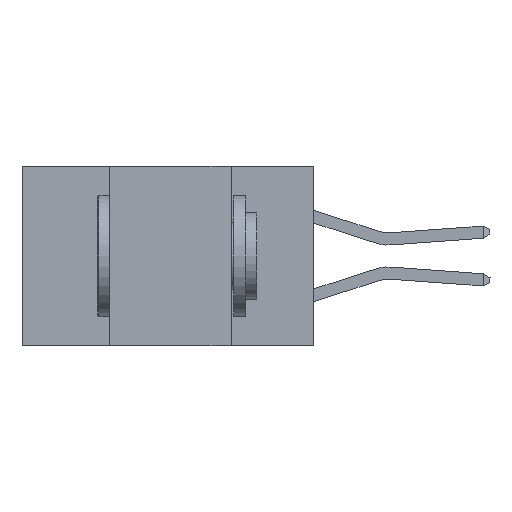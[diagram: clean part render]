
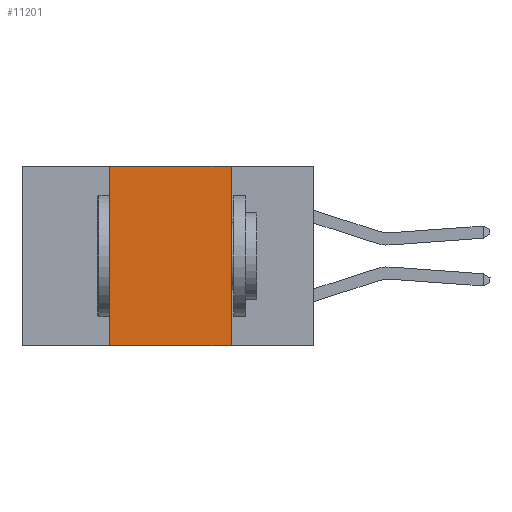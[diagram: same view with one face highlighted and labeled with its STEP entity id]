
A CAD part, left-side view. The second image highlights one B-rep face of the part: STEP entity #11201.
In plain terms, the highlighted planar face has unit normal (-1, 0, 0).
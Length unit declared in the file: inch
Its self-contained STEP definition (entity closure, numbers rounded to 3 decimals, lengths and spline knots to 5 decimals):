
#2424 = ORIENTED_EDGE ( 'NONE', *, *, #34790, .F. ) ;
#2858 = PLANE ( 'NONE',  #18497 ) ;
#3801 = ORIENTED_EDGE ( 'NONE', *, *, #26579, .F. ) ;
#4964 = LINE ( 'NONE', #28506, #28670 ) ;
#5660 = ORIENTED_EDGE ( 'NONE', *, *, #21838, .T. ) ;
#5968 = DIRECTION ( 'NONE',  ( 1., 0., 0. ) ) ;
#6004 = CARTESIAN_POINT ( 'NONE',  ( 0., 0.6, 0. ) ) ;
#9249 = DIRECTION ( 'NONE',  ( 0., -1., 0. ) ) ;
#9551 = FACE_OUTER_BOUND ( 'NONE', #30618, .T. ) ;
#10590 = CARTESIAN_POINT ( 'NONE',  ( 0., 0.42, 0. ) ) ;
#11201 = ADVANCED_FACE ( 'NONE', ( #9551 ), #2858, .F. ) ;
#11910 = LINE ( 'NONE', #6004, #27706 ) ;
#17812 = DIRECTION ( 'NONE',  ( 0., 0., 1. ) ) ;
#18471 = CARTESIAN_POINT ( 'NONE',  ( 0., 0.6, -0.37 ) ) ;
#18497 = AXIS2_PLACEMENT_3D ( 'NONE', #23271, #5968, #33219 ) ;
#18858 = LINE ( 'NONE', #10590, #33550 ) ;
#19615 = LINE ( 'NONE', #18471, #39555 ) ;
#20816 = VERTEX_POINT ( 'NONE', #38798 ) ;
#21838 = EDGE_CURVE ( 'NONE', #32432, #40290, #19615, .T. ) ;
#23271 = CARTESIAN_POINT ( 'NONE',  ( 0., 0.6, 0. ) ) ;
#25886 = EDGE_CURVE ( 'NONE', #35280, #20816, #11910, .T. ) ;
#26579 = EDGE_CURVE ( 'NONE', #20816, #40290, #4964, .T. ) ;
#27706 = VECTOR ( 'NONE', #9249, 39.37008 ) ;
#28506 = CARTESIAN_POINT ( 'NONE',  ( 0., 0.17, 0. ) ) ;
#28644 = DIRECTION ( 'NONE',  ( 0., 0., -1. ) ) ;
#28670 = VECTOR ( 'NONE', #28644, 39.37008 ) ;
#28706 = DIRECTION ( 'NONE',  ( 0., -1., 0. ) ) ;
#29503 = CARTESIAN_POINT ( 'NONE',  ( 0., 0.42, 0. ) ) ;
#30618 = EDGE_LOOP ( 'NONE', ( #3801, #35808, #2424, #5660 ) ) ;
#32432 = VERTEX_POINT ( 'NONE', #42501 ) ;
#33219 = DIRECTION ( 'NONE',  ( 0., 0., -1. ) ) ;
#33550 = VECTOR ( 'NONE', #17812, 39.37008 ) ;
#34790 = EDGE_CURVE ( 'NONE', #32432, #35280, #18858, .T. ) ;
#35280 = VERTEX_POINT ( 'NONE', #29503 ) ;
#35808 = ORIENTED_EDGE ( 'NONE', *, *, #25886, .F. ) ;
#37112 = CARTESIAN_POINT ( 'NONE',  ( 0., 0.17, -0.37 ) ) ;
#38798 = CARTESIAN_POINT ( 'NONE',  ( 0., 0.17, 0. ) ) ;
#39555 = VECTOR ( 'NONE', #28706, 39.37008 ) ;
#40290 = VERTEX_POINT ( 'NONE', #37112 ) ;
#42501 = CARTESIAN_POINT ( 'NONE',  ( 0., 0.42, -0.37 ) ) ;
